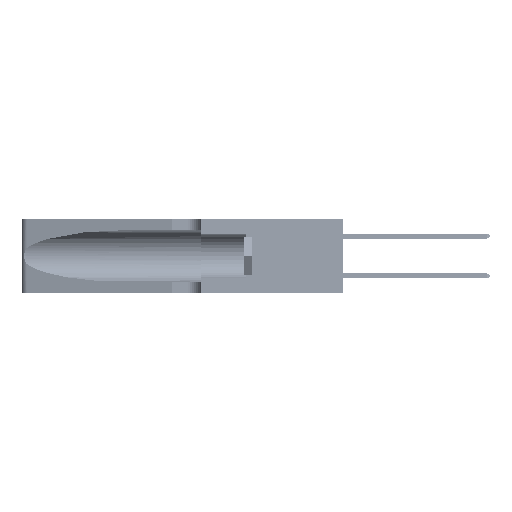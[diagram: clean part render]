
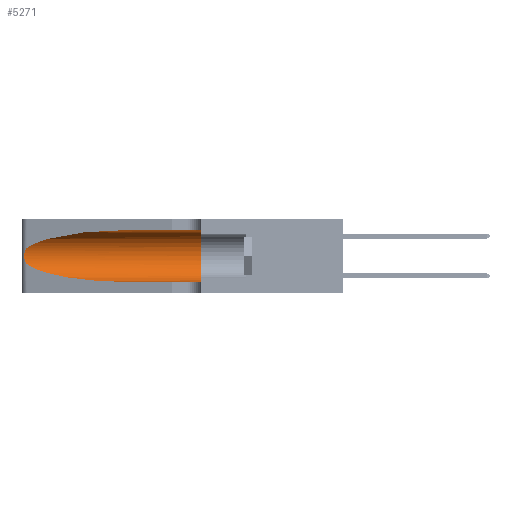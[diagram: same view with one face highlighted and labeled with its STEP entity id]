
A CAD part, left-side view. The second image highlights one B-rep face of the part: STEP entity #5271.
In plain terms, the highlighted cylindrical face has radius 3.308 mm (diameter 6.617 mm), a partial arc.
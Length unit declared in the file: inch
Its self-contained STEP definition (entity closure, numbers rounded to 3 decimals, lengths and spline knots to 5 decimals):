
#237 = EDGE_CURVE ( 'NONE', #15609, #28383, #32595, .T. ) ;
#600 = CARTESIAN_POINT ( 'NONE',  ( 0.25487, 1.22718, 0.22369 ) ) ;
#2165 = CARTESIAN_POINT ( 'NONE',  ( 0.25854, 1.2359, 0.20912 ) ) ;
#2824 = EDGE_CURVE ( 'NONE', #44166, #15609, #48911, .T. ) ;
#5271 = ADVANCED_FACE ( 'NONE', ( #23517 ), #26730, .F. ) ;
#5846 = DIRECTION ( 'NONE',  ( 0., 0., -1. ) ) ;
#5883 = CARTESIAN_POINT ( 'NONE',  ( 0.25487, 1.22718, 0.14631 ) ) ;
#6650 = CARTESIAN_POINT ( 'NONE',  ( 0.1305, 0.72297, 0.05475 ) ) ;
#6708 = CARTESIAN_POINT ( 'NONE',  ( 0.26017, 1.23833, 0.17102 ) ) ;
#8079 = ORIENTED_EDGE ( 'NONE', *, *, #237, .T. ) ;
#10520 = CARTESIAN_POINT ( 'NONE',  ( 0.25639, 1.23186, 0.15144 ) ) ;
#11969 = ORIENTED_EDGE ( 'NONE', *, *, #35244, .F. ) ;
#13109 = CARTESIAN_POINT ( 'NONE',  ( 0.1305, 0.72297, 0.31525 ) ) ;
#13446 = EDGE_CURVE ( 'NONE', #15252, #44883, #14819, .T. ) ;
#14132 =( BOUNDED_CURVE ( )  B_SPLINE_CURVE ( 3, ( #43824, #31639, #47991, #6650 ),
 .UNSPECIFIED., .F., .F. ) 
 B_SPLINE_CURVE_WITH_KNOTS ( ( 4, 4 ),
 ( 3.44316, 4.71239 ),
 .UNSPECIFIED. ) 
 CURVE ( )  GEOMETRIC_REPRESENTATION_ITEM ( )  RATIONAL_B_SPLINE_CURVE ( ( 1., 0.87, 0.87, 1. ) ) 
 REPRESENTATION_ITEM ( '' )  );
#14819 = LINE ( 'NONE', #41629, #15493 ) ;
#15041 = CARTESIAN_POINT ( 'NONE',  ( 0.25555, 1.22994, 0.2215 ) ) ;
#15214 = CARTESIAN_POINT ( 'NONE',  ( 0.25487, 1.22718, 0.22369 ) ) ;
#15252 = VERTEX_POINT ( 'NONE', #23503 ) ;
#15493 = VECTOR ( 'NONE', #33259, 39.37008 ) ;
#15609 = VERTEX_POINT ( 'NONE', #42047 ) ;
#17622 = CARTESIAN_POINT ( 'NONE',  ( 0.1305, 0.35, 0.05475 ) ) ;
#18690 = CARTESIAN_POINT ( 'NONE',  ( 0.25787, 1.23484, 0.2124 ) ) ;
#20218 = ORIENTED_EDGE ( 'NONE', *, *, #29094, .F. ) ;
#20271 = LINE ( 'NONE', #22748, #36674 ) ;
#22415 = CARTESIAN_POINT ( 'NONE',  ( 0.1305, 1.61858, 0.185 ) ) ;
#22748 = CARTESIAN_POINT ( 'NONE',  ( 0.1305, 1.61858, 0.31525 ) ) ;
#23110 = CARTESIAN_POINT ( 'NONE',  ( 0.25487, 1.22718, 0.14631 ) ) ;
#23503 = CARTESIAN_POINT ( 'NONE',  ( 0.1305, 0.72297, 0.05475 ) ) ;
#23506 = EDGE_LOOP ( 'NONE', ( #44120, #8079, #26608, #52235, #11969, #20218 ) ) ;
#23517 = FACE_OUTER_BOUND ( 'NONE', #23506, .T. ) ;
#26608 = ORIENTED_EDGE ( 'NONE', *, *, #44005, .T. ) ;
#26730 = CYLINDRICAL_SURFACE ( 'NONE', #52467, 0.13025 ) ;
#26941 = CARTESIAN_POINT ( 'NONE',  ( 0.26075, 1.23896, 0.178 ) ) ;
#27129 = CARTESIAN_POINT ( 'NONE',  ( 0.25639, 1.23184, 0.21858 ) ) ;
#28383 = VERTEX_POINT ( 'NONE', #5883 ) ;
#29094 = EDGE_CURVE ( 'NONE', #44166, #44039, #20271, .T. ) ;
#31139 = CARTESIAN_POINT ( 'NONE',  ( 0.25789, 1.23486, 0.15765 ) ) ;
#31335 = CARTESIAN_POINT ( 'NONE',  ( 0.25856, 1.23593, 0.16098 ) ) ;
#31639 = CARTESIAN_POINT ( 'NONE',  ( 0.2373, 1.15595, 0.08982 ) ) ;
#31692 = CARTESIAN_POINT ( 'NONE',  ( 0.26075, 1.23896, 0.19203 ) ) ;
#32303 = DIRECTION ( 'NONE',  ( 0., 0., 1. ) ) ;
#32595 = B_SPLINE_CURVE_WITH_KNOTS ( 'NONE', 3,
 ( #15214, #15041, #27129, #18690, #2165, #47694, #31692, #26941, #6708, #31335, #31139, #10520, #35365, #23110 ),
 .UNSPECIFIED., .F., .F.,
 ( 4, 2, 2, 2, 2, 2, 4 ),
 ( 0., 0.00027, 0.00053, 0.00107, 0.0016, 0.00187, 0.00214 ),
 .UNSPECIFIED. ) ;
#33259 = DIRECTION ( 'NONE',  ( 0., -1., 0. ) ) ;
#34976 = AXIS2_PLACEMENT_3D ( 'NONE', #53748, #53212, #32303 ) ;
#35244 = EDGE_CURVE ( 'NONE', #44039, #44883, #51935, .T. ) ;
#35365 = CARTESIAN_POINT ( 'NONE',  ( 0.25555, 1.22993, 0.14849 ) ) ;
#36674 = VECTOR ( 'NONE', #40454, 39.37008 ) ;
#40454 = DIRECTION ( 'NONE',  ( 0., -1., 0. ) ) ;
#41629 = CARTESIAN_POINT ( 'NONE',  ( 0.1305, 1.61858, 0.05475 ) ) ;
#42047 = CARTESIAN_POINT ( 'NONE',  ( 0.25487, 1.22718, 0.22369 ) ) ;
#43824 = CARTESIAN_POINT ( 'NONE',  ( 0.25487, 1.22718, 0.14631 ) ) ;
#44005 = EDGE_CURVE ( 'NONE', #28383, #15252, #14132, .T. ) ;
#44039 = VERTEX_POINT ( 'NONE', #49243 ) ;
#44120 = ORIENTED_EDGE ( 'NONE', *, *, #2824, .T. ) ;
#44166 = VERTEX_POINT ( 'NONE', #45243 ) ;
#44883 = VERTEX_POINT ( 'NONE', #17622 ) ;
#45243 = CARTESIAN_POINT ( 'NONE',  ( 0.1305, 0.72297, 0.31525 ) ) ;
#47694 = CARTESIAN_POINT ( 'NONE',  ( 0.26018, 1.23835, 0.19895 ) ) ;
#47991 = CARTESIAN_POINT ( 'NONE',  ( 0.18966, 0.96281, 0.05475 ) ) ;
#48911 =( BOUNDED_CURVE ( )  B_SPLINE_CURVE ( 3, ( #13109, #50689, #50501, #600 ),
 .UNSPECIFIED., .F., .F. ) 
 B_SPLINE_CURVE_WITH_KNOTS ( ( 4, 4 ),
 ( 1.5708, 2.84003 ),
 .UNSPECIFIED. ) 
 CURVE ( )  GEOMETRIC_REPRESENTATION_ITEM ( )  RATIONAL_B_SPLINE_CURVE ( ( 1., 0.87, 0.87, 1. ) ) 
 REPRESENTATION_ITEM ( '' )  );
#49243 = CARTESIAN_POINT ( 'NONE',  ( 0.1305, 0.35, 0.31525 ) ) ;
#50501 = CARTESIAN_POINT ( 'NONE',  ( 0.2373, 1.15595, 0.28018 ) ) ;
#50689 = CARTESIAN_POINT ( 'NONE',  ( 0.18966, 0.96281, 0.31525 ) ) ;
#51565 = DIRECTION ( 'NONE',  ( 0., -1., 0. ) ) ;
#51935 = CIRCLE ( 'NONE', #34976, 0.13025 ) ;
#52235 = ORIENTED_EDGE ( 'NONE', *, *, #13446, .T. ) ;
#52467 = AXIS2_PLACEMENT_3D ( 'NONE', #22415, #51565, #5846 ) ;
#53212 = DIRECTION ( 'NONE',  ( 0., 1., 0. ) ) ;
#53748 = CARTESIAN_POINT ( 'NONE',  ( 0.1305, 0.35, 0.185 ) ) ;
